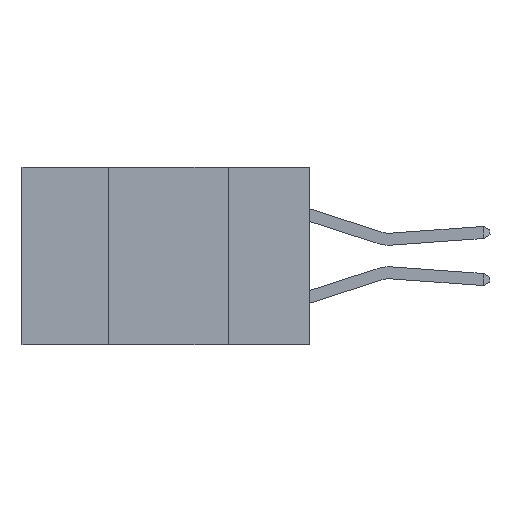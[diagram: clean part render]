
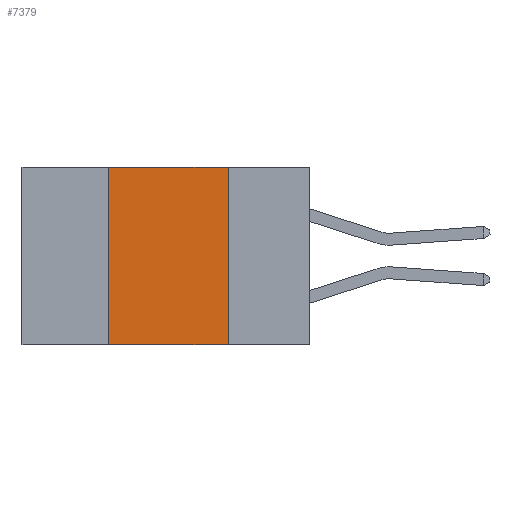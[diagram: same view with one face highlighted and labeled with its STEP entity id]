
A CAD part, left-side view. The second image highlights one B-rep face of the part: STEP entity #7379.
In plain terms, the highlighted planar face has unit normal (-1, 0, 0).
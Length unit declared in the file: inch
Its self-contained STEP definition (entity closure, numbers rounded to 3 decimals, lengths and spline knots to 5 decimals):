
#315 = VECTOR ( 'NONE', #10065, 39.37008 ) ;
#398 = EDGE_CURVE ( 'NONE', #3270, #9142, #7043, .T. ) ;
#711 = FACE_OUTER_BOUND ( 'NONE', #10142, .T. ) ;
#898 = DIRECTION ( 'NONE',  ( 0., 0., 1. ) ) ;
#2397 = EDGE_CURVE ( 'NONE', #9142, #6957, #4389, .T. ) ;
#3270 = VERTEX_POINT ( 'NONE', #3934 ) ;
#3372 = VECTOR ( 'NONE', #898, 39.37008 ) ;
#3739 = CARTESIAN_POINT ( 'NONE',  ( 0., 0.17, 0. ) ) ;
#3747 = VERTEX_POINT ( 'NONE', #7131 ) ;
#3934 = CARTESIAN_POINT ( 'NONE',  ( 0., 0.42, 0. ) ) ;
#4389 = LINE ( 'NONE', #3739, #10430 ) ;
#4606 = CARTESIAN_POINT ( 'NONE',  ( 0., 0.17, -0.37 ) ) ;
#4615 = EDGE_CURVE ( 'NONE', #3747, #3270, #9962, .T. ) ;
#5138 = CARTESIAN_POINT ( 'NONE',  ( 0., 0.6, -0.37 ) ) ;
#5153 = DIRECTION ( 'NONE',  ( 0., 0., -1. ) ) ;
#5975 = CARTESIAN_POINT ( 'NONE',  ( 0., 0.6, 0. ) ) ;
#6334 = ORIENTED_EDGE ( 'NONE', *, *, #8033, .T. ) ;
#6957 = VERTEX_POINT ( 'NONE', #4606 ) ;
#6975 = ORIENTED_EDGE ( 'NONE', *, *, #398, .F. ) ;
#7043 = LINE ( 'NONE', #9707, #9231 ) ;
#7131 = CARTESIAN_POINT ( 'NONE',  ( 0., 0.42, -0.37 ) ) ;
#7238 = CARTESIAN_POINT ( 'NONE',  ( 0., 0.42, 0. ) ) ;
#7379 = ADVANCED_FACE ( 'NONE', ( #711 ), #8446, .F. ) ;
#8033 = EDGE_CURVE ( 'NONE', #3747, #6957, #8903, .T. ) ;
#8446 = PLANE ( 'NONE',  #8551 ) ;
#8515 = DIRECTION ( 'NONE',  ( 0., 0., -1. ) ) ;
#8551 = AXIS2_PLACEMENT_3D ( 'NONE', #5975, #10077, #5153 ) ;
#8903 = LINE ( 'NONE', #5138, #315 ) ;
#8934 = DIRECTION ( 'NONE',  ( 0., -1., 0. ) ) ;
#9142 = VERTEX_POINT ( 'NONE', #10124 ) ;
#9231 = VECTOR ( 'NONE', #8934, 39.37008 ) ;
#9405 = ORIENTED_EDGE ( 'NONE', *, *, #4615, .F. ) ;
#9707 = CARTESIAN_POINT ( 'NONE',  ( 0., 0.6, 0. ) ) ;
#9962 = LINE ( 'NONE', #7238, #3372 ) ;
#10065 = DIRECTION ( 'NONE',  ( 0., -1., 0. ) ) ;
#10077 = DIRECTION ( 'NONE',  ( 1., 0., 0. ) ) ;
#10124 = CARTESIAN_POINT ( 'NONE',  ( 0., 0.17, 0. ) ) ;
#10142 = EDGE_LOOP ( 'NONE', ( #10280, #6975, #9405, #6334 ) ) ;
#10280 = ORIENTED_EDGE ( 'NONE', *, *, #2397, .F. ) ;
#10430 = VECTOR ( 'NONE', #8515, 39.37008 ) ;
